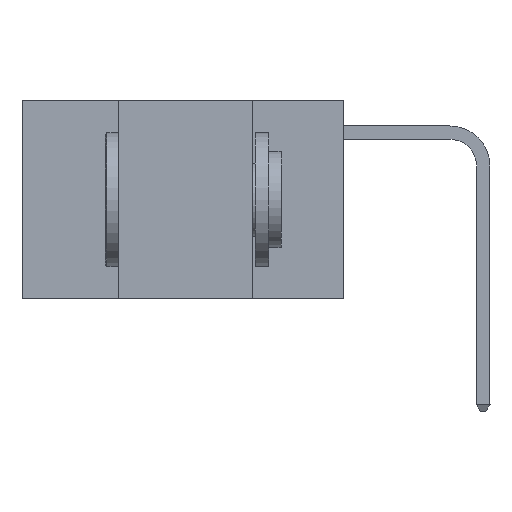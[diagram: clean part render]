
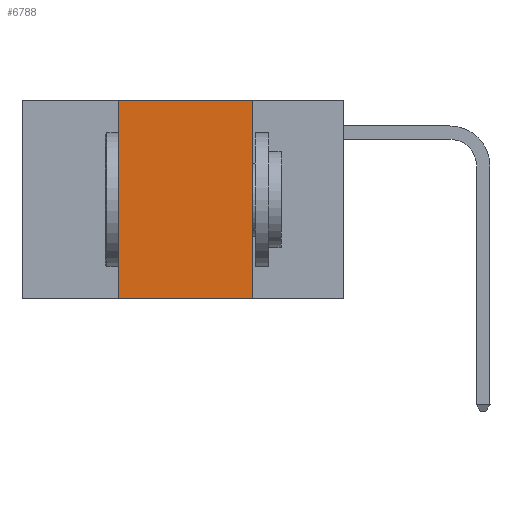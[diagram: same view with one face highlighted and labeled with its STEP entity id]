
A CAD part, left-side view. The second image highlights one B-rep face of the part: STEP entity #6788.
In plain terms, the highlighted planar face has unit normal (-1, 0, 0).
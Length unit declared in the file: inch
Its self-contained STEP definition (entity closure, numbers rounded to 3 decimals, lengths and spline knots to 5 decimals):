
#15 = VECTOR ( 'NONE', #11248, 39.37008 ) ;
#105 = VERTEX_POINT ( 'NONE', #19178 ) ;
#292 = ORIENTED_EDGE ( 'NONE', *, *, #20419, .T. ) ;
#608 = LINE ( 'NONE', #9806, #2697 ) ;
#721 = ORIENTED_EDGE ( 'NONE', *, *, #15947, .F. ) ;
#759 = DIRECTION ( 'NONE',  ( 0., 0., -1. ) ) ;
#2052 = CARTESIAN_POINT ( 'NONE',  ( 0., 0.6, 0. ) ) ;
#2493 = DIRECTION ( 'NONE',  ( 0., 0., -1. ) ) ;
#2697 = VECTOR ( 'NONE', #759, 39.37008 ) ;
#2698 = EDGE_CURVE ( 'NONE', #9007, #27877, #20161, .T. ) ;
#4603 = FACE_OUTER_BOUND ( 'NONE', #25446, .T. ) ;
#6242 = VECTOR ( 'NONE', #11392, 39.37008 ) ;
#6788 = ADVANCED_FACE ( 'NONE', ( #4603 ), #21058, .F. ) ;
#7003 = CARTESIAN_POINT ( 'NONE',  ( 0., 0.6, 0. ) ) ;
#7100 = AXIS2_PLACEMENT_3D ( 'NONE', #7003, #11546, #2493 ) ;
#9007 = VERTEX_POINT ( 'NONE', #9815 ) ;
#9120 = CARTESIAN_POINT ( 'NONE',  ( 0., 0.42, 0. ) ) ;
#9806 = CARTESIAN_POINT ( 'NONE',  ( 0., 0.17, 0. ) ) ;
#9815 = CARTESIAN_POINT ( 'NONE',  ( 0., 0.42, 0. ) ) ;
#11248 = DIRECTION ( 'NONE',  ( 0., -1., 0. ) ) ;
#11392 = DIRECTION ( 'NONE',  ( 0., 0., 1. ) ) ;
#11396 = DIRECTION ( 'NONE',  ( 0., -1., 0. ) ) ;
#11546 = DIRECTION ( 'NONE',  ( 1., 0., 0. ) ) ;
#11975 = CARTESIAN_POINT ( 'NONE',  ( 0., 0.17, 0. ) ) ;
#13058 = CARTESIAN_POINT ( 'NONE',  ( 0., 0.6, -0.37 ) ) ;
#15947 = EDGE_CURVE ( 'NONE', #27877, #21898, #608, .T. ) ;
#16377 = LINE ( 'NONE', #9120, #6242 ) ;
#18064 = CARTESIAN_POINT ( 'NONE',  ( 0., 0.17, -0.37 ) ) ;
#19178 = CARTESIAN_POINT ( 'NONE',  ( 0., 0.42, -0.37 ) ) ;
#20161 = LINE ( 'NONE', #2052, #26838 ) ;
#20419 = EDGE_CURVE ( 'NONE', #105, #21898, #27234, .T. ) ;
#20668 = EDGE_CURVE ( 'NONE', #105, #9007, #16377, .T. ) ;
#21058 = PLANE ( 'NONE',  #7100 ) ;
#21898 = VERTEX_POINT ( 'NONE', #18064 ) ;
#23483 = ORIENTED_EDGE ( 'NONE', *, *, #2698, .F. ) ;
#25446 = EDGE_LOOP ( 'NONE', ( #721, #23483, #27110, #292 ) ) ;
#26838 = VECTOR ( 'NONE', #11396, 39.37008 ) ;
#27110 = ORIENTED_EDGE ( 'NONE', *, *, #20668, .F. ) ;
#27234 = LINE ( 'NONE', #13058, #15 ) ;
#27877 = VERTEX_POINT ( 'NONE', #11975 ) ;
